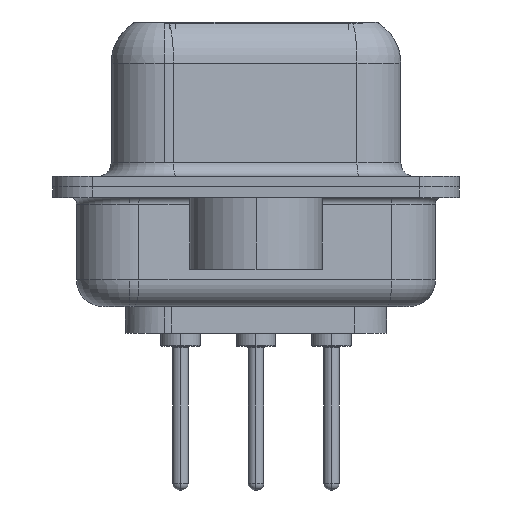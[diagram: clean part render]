
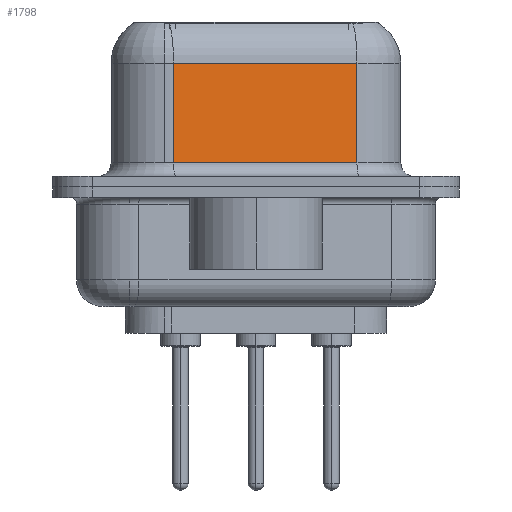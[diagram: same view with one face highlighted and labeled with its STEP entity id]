
A CAD part, left-side view. The second image highlights one B-rep face of the part: STEP entity #1798.
In plain terms, the highlighted planar face has unit normal (-0.985, -0.174, 0).
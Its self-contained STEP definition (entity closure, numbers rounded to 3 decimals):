
#771 = CARTESIAN_POINT ( 'NONE',  ( 5.647, -3.797, 6.4 ) ) ;
#1798 = ADVANCED_FACE ( 'NONE', ( #23377 ), #8143, .F. ) ;
#2069 = EDGE_CURVE ( 'NONE', #32699, #24675, #9956, .T. ) ;
#2192 = ORIENTED_EDGE ( 'NONE', *, *, #9918, .T. ) ;
#2300 = VERTEX_POINT ( 'NONE', #23686 ) ;
#3362 = ORIENTED_EDGE ( 'NONE', *, *, #13788, .T. ) ;
#6475 = VECTOR ( 'NONE', #12899, 1000. ) ;
#6482 = EDGE_LOOP ( 'NONE', ( #21410, #2192, #30355, #3362 ) ) ;
#8079 = LINE ( 'NONE', #18306, #30504 ) ;
#8143 = PLANE ( 'NONE',  #16431 ) ;
#9397 = VERTEX_POINT ( 'NONE', #10647 ) ;
#9918 = EDGE_CURVE ( 'NONE', #32699, #2300, #8079, .T. ) ;
#9956 = LINE ( 'NONE', #22368, #31914 ) ;
#10647 = CARTESIAN_POINT ( 'NONE',  ( 4.43, 3.103, 0.9 ) ) ;
#12899 = DIRECTION ( 'NONE',  ( 0.174, -0.985, 0. ) ) ;
#13322 = DIRECTION ( 'NONE',  ( 0.985, 0.174, 0. ) ) ;
#13749 = LINE ( 'NONE', #21474, #30456 ) ;
#13788 = EDGE_CURVE ( 'NONE', #9397, #24675, #24870, .T. ) ;
#14677 = DIRECTION ( 'NONE',  ( 0., 0., -1. ) ) ;
#16431 = AXIS2_PLACEMENT_3D ( 'NONE', #771, #13322, #28875 ) ;
#18306 = CARTESIAN_POINT ( 'NONE',  ( 5.647, -3.797, 4.65 ) ) ;
#21410 = ORIENTED_EDGE ( 'NONE', *, *, #2069, .F. ) ;
#21474 = CARTESIAN_POINT ( 'NONE',  ( 4.43, 3.103, 6.4 ) ) ;
#22260 = EDGE_CURVE ( 'NONE', #2300, #9397, #13749, .T. ) ;
#22368 = CARTESIAN_POINT ( 'NONE',  ( 5.647, -3.797, 6.4 ) ) ;
#23377 = FACE_OUTER_BOUND ( 'NONE', #6482, .T. ) ;
#23686 = CARTESIAN_POINT ( 'NONE',  ( 4.43, 3.103, 4.65 ) ) ;
#24675 = VERTEX_POINT ( 'NONE', #26135 ) ;
#24870 = LINE ( 'NONE', #30457, #6475 ) ;
#25843 = DIRECTION ( 'NONE',  ( -0.174, 0.985, 0. ) ) ;
#26135 = CARTESIAN_POINT ( 'NONE',  ( 5.647, -3.797, 0.9 ) ) ;
#28875 = DIRECTION ( 'NONE',  ( -0.174, 0.985, 0. ) ) ;
#30355 = ORIENTED_EDGE ( 'NONE', *, *, #22260, .T. ) ;
#30456 = VECTOR ( 'NONE', #31622, 1000. ) ;
#30457 = CARTESIAN_POINT ( 'NONE',  ( 5.647, -3.797, 0.9 ) ) ;
#30504 = VECTOR ( 'NONE', #25843, 1000. ) ;
#31622 = DIRECTION ( 'NONE',  ( 0., 0., -1. ) ) ;
#31914 = VECTOR ( 'NONE', #14677, 1000. ) ;
#32672 = CARTESIAN_POINT ( 'NONE',  ( 5.647, -3.797, 4.65 ) ) ;
#32699 = VERTEX_POINT ( 'NONE', #32672 ) ;
